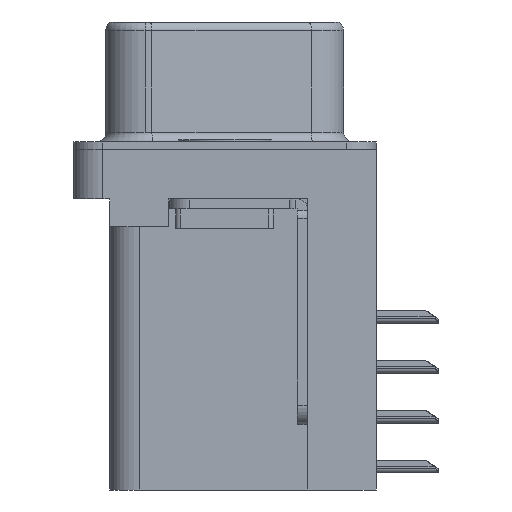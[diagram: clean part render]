
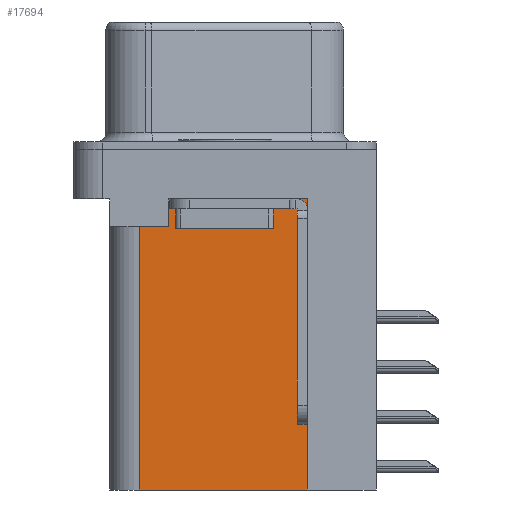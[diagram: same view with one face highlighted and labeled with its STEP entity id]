
A CAD part, left-side view. The second image highlights one B-rep face of the part: STEP entity #17694.
In plain terms, the highlighted planar face has unit normal (-1, 0, 0).
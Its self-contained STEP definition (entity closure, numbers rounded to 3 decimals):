
#139 = EDGE_CURVE ( 'NONE', #26102, #23779, #21150, .T. ) ;
#2658 = EDGE_CURVE ( 'NONE', #7238, #8252, #26835, .T. ) ;
#2672 = CARTESIAN_POINT ( 'NONE',  ( 3.75, -4.2, -17.3 ) ) ;
#2750 = CARTESIAN_POINT ( 'NONE',  ( 3.75, -4.2, -17.3 ) ) ;
#3094 = DIRECTION ( 'NONE',  ( 0., 0., 1. ) ) ;
#4067 = ORIENTED_EDGE ( 'NONE', *, *, #16932, .F. ) ;
#4166 = DIRECTION ( 'NONE',  ( 0., 0., -1. ) ) ;
#4313 = LINE ( 'NONE', #27072, #17404 ) ;
#7238 = VERTEX_POINT ( 'NONE', #15921 ) ;
#8252 = VERTEX_POINT ( 'NONE', #8788 ) ;
#8377 = CARTESIAN_POINT ( 'NONE',  ( 3.75, -4.2, -2.5 ) ) ;
#8788 = CARTESIAN_POINT ( 'NONE',  ( 3.75, -4.2, -2.5 ) ) ;
#10188 = LINE ( 'NONE', #8377, #25270 ) ;
#10608 = VECTOR ( 'NONE', #4166, 1000. ) ;
#13007 = DIRECTION ( 'NONE',  ( 0., 1., 0. ) ) ;
#13154 = CARTESIAN_POINT ( 'NONE',  ( 3.75, 2.85, -3.9 ) ) ;
#13805 = ORIENTED_EDGE ( 'NONE', *, *, #27334, .T. ) ;
#13892 = FACE_OUTER_BOUND ( 'NONE', #16779, .T. ) ;
#14629 = VERTEX_POINT ( 'NONE', #24507 ) ;
#15634 = CARTESIAN_POINT ( 'NONE',  ( 3.75, 4.35, -3.9 ) ) ;
#15921 = CARTESIAN_POINT ( 'NONE',  ( 3.75, -4.2, -17.3 ) ) ;
#16255 = EDGE_CURVE ( 'NONE', #8252, #14629, #10188, .T. ) ;
#16779 = EDGE_LOOP ( 'NONE', ( #33005, #13805, #27392, #27376, #4067, #19620 ) ) ;
#16932 = EDGE_CURVE ( 'NONE', #7238, #28375, #17656, .T. ) ;
#17404 = VECTOR ( 'NONE', #3094, 1000. ) ;
#17656 = LINE ( 'NONE', #2750, #24756 ) ;
#17694 = ADVANCED_FACE ( 'NONE', ( #13892 ), #22022, .F. ) ;
#19620 = ORIENTED_EDGE ( 'NONE', *, *, #2658, .T. ) ;
#19949 = DIRECTION ( 'NONE',  ( 0., 1., 0. ) ) ;
#21123 = VECTOR ( 'NONE', #19949, 1000. ) ;
#21150 = LINE ( 'NONE', #22732, #21123 ) ;
#22022 = PLANE ( 'NONE',  #27731 ) ;
#22732 = CARTESIAN_POINT ( 'NONE',  ( 3.75, 0., -3.9 ) ) ;
#23771 = DIRECTION ( 'NONE',  ( 0., 1., 0. ) ) ;
#23779 = VERTEX_POINT ( 'NONE', #15634 ) ;
#24507 = CARTESIAN_POINT ( 'NONE',  ( 3.75, 2.85, -2.5 ) ) ;
#24756 = VECTOR ( 'NONE', #23771, 1000. ) ;
#24898 = CARTESIAN_POINT ( 'NONE',  ( 3.75, 4.35, -17.3 ) ) ;
#25270 = VECTOR ( 'NONE', #35537, 1000. ) ;
#26102 = VERTEX_POINT ( 'NONE', #37645 ) ;
#26532 = VECTOR ( 'NONE', #29451, 1000. ) ;
#26835 = LINE ( 'NONE', #2672, #26532 ) ;
#27072 = CARTESIAN_POINT ( 'NONE',  ( 3.75, 4.35, -17.3 ) ) ;
#27334 = EDGE_CURVE ( 'NONE', #14629, #26102, #33684, .T. ) ;
#27376 = ORIENTED_EDGE ( 'NONE', *, *, #38437, .F. ) ;
#27392 = ORIENTED_EDGE ( 'NONE', *, *, #139, .T. ) ;
#27731 = AXIS2_PLACEMENT_3D ( 'NONE', #27986, #30975, #13007 ) ;
#27986 = CARTESIAN_POINT ( 'NONE',  ( 3.75, -4.2, -17.3 ) ) ;
#28375 = VERTEX_POINT ( 'NONE', #24898 ) ;
#29451 = DIRECTION ( 'NONE',  ( 0., 0., 1. ) ) ;
#30975 = DIRECTION ( 'NONE',  ( 1., 0., 0. ) ) ;
#33005 = ORIENTED_EDGE ( 'NONE', *, *, #16255, .T. ) ;
#33684 = LINE ( 'NONE', #13154, #10608 ) ;
#35537 = DIRECTION ( 'NONE',  ( 0., 1., 0. ) ) ;
#37645 = CARTESIAN_POINT ( 'NONE',  ( 3.75, 2.85, -3.9 ) ) ;
#38437 = EDGE_CURVE ( 'NONE', #28375, #23779, #4313, .T. ) ;
